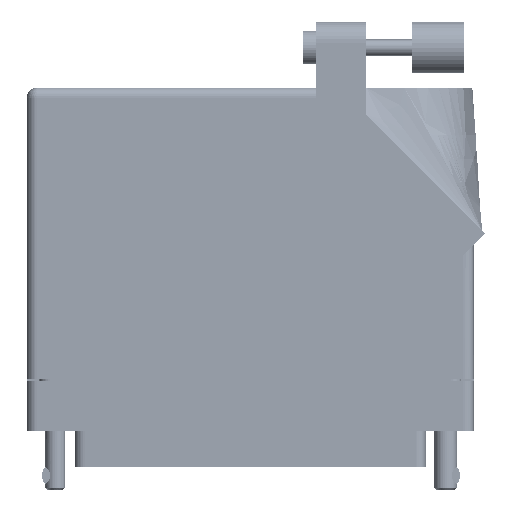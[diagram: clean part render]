
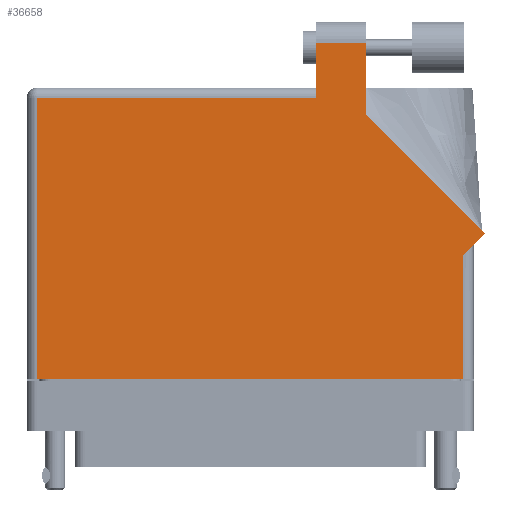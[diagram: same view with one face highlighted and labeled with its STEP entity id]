
A CAD part, front view. The second image highlights one B-rep face of the part: STEP entity #36658.
In plain terms, the highlighted face is planar.
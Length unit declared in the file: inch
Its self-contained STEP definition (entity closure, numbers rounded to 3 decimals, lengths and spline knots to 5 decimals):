
#2601 = VERTEX_POINT ( 'NONE', #53037 ) ;
#3620 = DIRECTION ( 'NONE',  ( 0.707, 0.707, 0. ) ) ;
#4361 = CARTESIAN_POINT ( 'NONE',  ( 0.399, 1.95, 0.617 ) ) ;
#5752 = PLANE ( 'NONE',  #68192 ) ;
#6437 = VECTOR ( 'NONE', #35678, 39.37008 ) ;
#7945 = DIRECTION ( 'NONE',  ( 0., 1., 0. ) ) ;
#7946 = EDGE_CURVE ( 'NONE', #30749, #72280, #74093, .T. ) ;
#8183 = LINE ( 'NONE', #36124, #15274 ) ;
#8245 = CARTESIAN_POINT ( 'NONE',  ( -1.297, -0.1, 0.617 ) ) ;
#10413 = CARTESIAN_POINT ( 'NONE',  ( 1.297, -0.1, 0.617 ) ) ;
#11623 = ORIENTED_EDGE ( 'NONE', *, *, #54603, .T. ) ;
#12294 = CARTESIAN_POINT ( 'NONE',  ( 1.297, 0.715, 0.617 ) ) ;
#13103 = CARTESIAN_POINT ( 'NONE',  ( -1.359, 1.675, 0.617 ) ) ;
#15274 = VECTOR ( 'NONE', #3620, 39.37008 ) ;
#17617 = LINE ( 'NONE', #67766, #6437 ) ;
#17691 = DIRECTION ( 'NONE',  ( -1., 0., 0. ) ) ;
#17710 = CARTESIAN_POINT ( 'NONE',  ( 0.399, 1.675, 0.617 ) ) ;
#19350 = DIRECTION ( 'NONE',  ( 0., 1., 0. ) ) ;
#21588 = ORIENTED_EDGE ( 'NONE', *, *, #40085, .T. ) ;
#22041 = VECTOR ( 'NONE', #7945, 39.37008 ) ;
#24228 = LINE ( 'NONE', #17710, #40383 ) ;
#29147 = FACE_OUTER_BOUND ( 'NONE', #60919, .T. ) ;
#30749 = VERTEX_POINT ( 'NONE', #58258 ) ;
#31340 = EDGE_CURVE ( 'NONE', #2601, #60708, #17617, .T. ) ;
#32362 = CARTESIAN_POINT ( 'NONE',  ( -1.297, 1.613, 0.617 ) ) ;
#35158 = LINE ( 'NONE', #79936, #22041 ) ;
#35591 = ORIENTED_EDGE ( 'NONE', *, *, #40780, .T. ) ;
#35678 = DIRECTION ( 'NONE',  ( 1., 0., 0. ) ) ;
#36124 = CARTESIAN_POINT ( 'NONE',  ( 1.359, 0.715, 0.617 ) ) ;
#36312 = ORIENTED_EDGE ( 'NONE', *, *, #7946, .T. ) ;
#36658 = ADVANCED_FACE ( 'NONE', ( #29147 ), #5752, .F. ) ;
#38105 = CARTESIAN_POINT ( 'NONE',  ( 0.399, 1.613, 0.617 ) ) ;
#38589 = EDGE_CURVE ( 'NONE', #39859, #2601, #73528, .T. ) ;
#38746 = CARTESIAN_POINT ( 'NONE',  ( -1.359, 1.613, 0.617 ) ) ;
#39144 = DIRECTION ( 'NONE',  ( 0., 0., -1. ) ) ;
#39859 = VERTEX_POINT ( 'NONE', #32362 ) ;
#40085 = EDGE_CURVE ( 'NONE', #60708, #67471, #71238, .T. ) ;
#40383 = VECTOR ( 'NONE', #82004, 39.37008 ) ;
#40780 = EDGE_CURVE ( 'NONE', #58745, #69476, #80270, .T. ) ;
#42088 = LINE ( 'NONE', #38746, #75625 ) ;
#45425 = CARTESIAN_POINT ( 'NONE',  ( 0.706, 1.50942, 0.617 ) ) ;
#47612 = DIRECTION ( 'NONE',  ( 0., -1., 0. ) ) ;
#48126 = VECTOR ( 'NONE', #47612, 39.37008 ) ;
#48223 = CARTESIAN_POINT ( 'NONE',  ( 1.42971, 0.78571, 0.617 ) ) ;
#50614 = ORIENTED_EDGE ( 'NONE', *, *, #31340, .T. ) ;
#53037 = CARTESIAN_POINT ( 'NONE',  ( -1.297, -0.1, 0.617 ) ) ;
#54603 = EDGE_CURVE ( 'NONE', #70342, #39859, #42088, .T. ) ;
#56786 = CARTESIAN_POINT ( 'NONE',  ( 0.706, 1.95, 0.617 ) ) ;
#58258 = CARTESIAN_POINT ( 'NONE',  ( 1.42971, 0.78571, 0.617 ) ) ;
#58745 = VERTEX_POINT ( 'NONE', #56786 ) ;
#60708 = VERTEX_POINT ( 'NONE', #10413 ) ;
#60919 = EDGE_LOOP ( 'NONE', ( #66217, #35591, #63622, #11623, #73781, #50614, #21588, #62237, #36312 ) ) ;
#61217 = EDGE_CURVE ( 'NONE', #69476, #70342, #24228, .T. ) ;
#62237 = ORIENTED_EDGE ( 'NONE', *, *, #64760, .T. ) ;
#63622 = ORIENTED_EDGE ( 'NONE', *, *, #61217, .T. ) ;
#64227 = DIRECTION ( 'NONE',  ( -1., 0., 0. ) ) ;
#64340 = CARTESIAN_POINT ( 'NONE',  ( 1.297, 0.653, 0.617 ) ) ;
#64760 = EDGE_CURVE ( 'NONE', #67471, #30749, #8183, .T. ) ;
#66217 = ORIENTED_EDGE ( 'NONE', *, *, #74508, .T. ) ;
#66588 = CARTESIAN_POINT ( 'NONE',  ( 0.399, 1.95, 0.617 ) ) ;
#67471 = VERTEX_POINT ( 'NONE', #64340 ) ;
#67766 = CARTESIAN_POINT ( 'NONE',  ( -1.359, -0.1, 0.617 ) ) ;
#68192 = AXIS2_PLACEMENT_3D ( 'NONE', #13103, #39144, #83925 ) ;
#69476 = VERTEX_POINT ( 'NONE', #66588 ) ;
#70342 = VERTEX_POINT ( 'NONE', #38105 ) ;
#71238 = LINE ( 'NONE', #12294, #74248 ) ;
#72280 = VERTEX_POINT ( 'NONE', #45425 ) ;
#73528 = LINE ( 'NONE', #8245, #48126 ) ;
#73781 = ORIENTED_EDGE ( 'NONE', *, *, #38589, .T. ) ;
#74093 = LINE ( 'NONE', #48223, #76129 ) ;
#74248 = VECTOR ( 'NONE', #19350, 39.37008 ) ;
#74508 = EDGE_CURVE ( 'NONE', #72280, #58745, #35158, .T. ) ;
#75625 = VECTOR ( 'NONE', #64227, 39.37008 ) ;
#76129 = VECTOR ( 'NONE', #79717, 39.37008 ) ;
#78137 = VECTOR ( 'NONE', #17691, 39.37008 ) ;
#79717 = DIRECTION ( 'NONE',  ( -0.707, 0.707, 0. ) ) ;
#79936 = CARTESIAN_POINT ( 'NONE',  ( 0.706, 1.50942, 0.617 ) ) ;
#80270 = LINE ( 'NONE', #4361, #78137 ) ;
#82004 = DIRECTION ( 'NONE',  ( 0., -1., 0. ) ) ;
#83925 = DIRECTION ( 'NONE',  ( -1., 0., 0. ) ) ;
